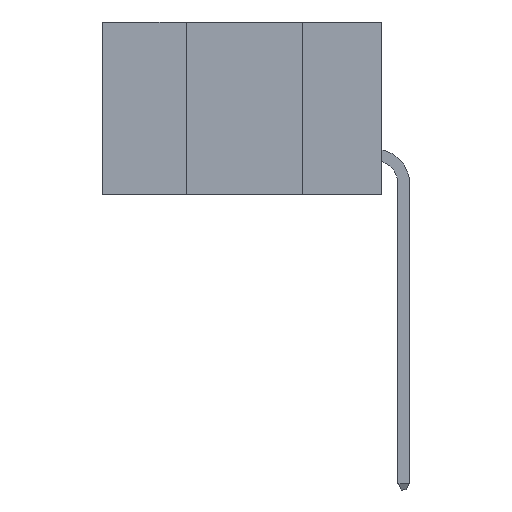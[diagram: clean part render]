
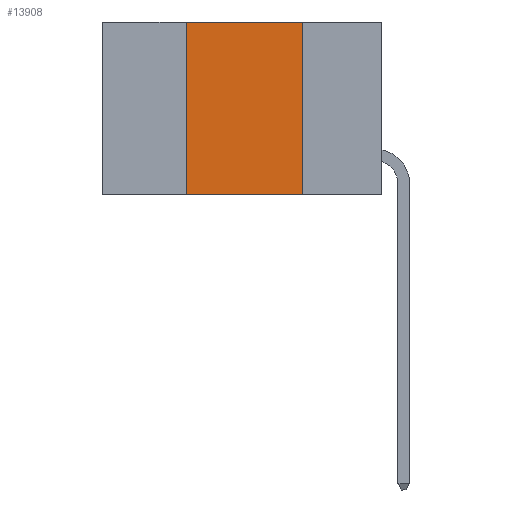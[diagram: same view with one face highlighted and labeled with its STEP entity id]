
A CAD part, left-side view. The second image highlights one B-rep face of the part: STEP entity #13908.
In plain terms, the highlighted planar face has unit normal (-1, 0, 0).
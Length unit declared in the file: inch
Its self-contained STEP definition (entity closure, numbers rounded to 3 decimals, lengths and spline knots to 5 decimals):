
#255 = LINE ( 'NONE', #19461, #16417 ) ;
#271 = EDGE_CURVE ( 'NONE', #3224, #4547, #255, .T. ) ;
#298 = ORIENTED_EDGE ( 'NONE', *, *, #18819, .F. ) ;
#656 = LINE ( 'NONE', #2862, #17238 ) ;
#894 = VERTEX_POINT ( 'NONE', #2922 ) ;
#2625 = AXIS2_PLACEMENT_3D ( 'NONE', #12504, #4800, #15581 ) ;
#2862 = CARTESIAN_POINT ( 'NONE',  ( 0., 0.42, 0. ) ) ;
#2922 = CARTESIAN_POINT ( 'NONE',  ( 0., 0.42, -0.37 ) ) ;
#3003 = DIRECTION ( 'NONE',  ( 0., -1., 0. ) ) ;
#3224 = VERTEX_POINT ( 'NONE', #3853 ) ;
#3259 = CARTESIAN_POINT ( 'NONE',  ( 0., 0.17, -0.37 ) ) ;
#3853 = CARTESIAN_POINT ( 'NONE',  ( 0., 0.42, 0. ) ) ;
#4547 = VERTEX_POINT ( 'NONE', #10092 ) ;
#4800 = DIRECTION ( 'NONE',  ( 1., 0., 0. ) ) ;
#4861 = EDGE_CURVE ( 'NONE', #4547, #14639, #5913, .T. ) ;
#5913 = LINE ( 'NONE', #13743, #10089 ) ;
#7158 = ORIENTED_EDGE ( 'NONE', *, *, #8276, .T. ) ;
#8276 = EDGE_CURVE ( 'NONE', #894, #14639, #17342, .T. ) ;
#9181 = DIRECTION ( 'NONE',  ( 0., 0., -1. ) ) ;
#9233 = ORIENTED_EDGE ( 'NONE', *, *, #4861, .F. ) ;
#9262 = VECTOR ( 'NONE', #3003, 39.37008 ) ;
#9538 = CARTESIAN_POINT ( 'NONE',  ( 0., 0.6, -0.37 ) ) ;
#10089 = VECTOR ( 'NONE', #9181, 39.37008 ) ;
#10092 = CARTESIAN_POINT ( 'NONE',  ( 0., 0.17, 0. ) ) ;
#10672 = ORIENTED_EDGE ( 'NONE', *, *, #271, .F. ) ;
#12504 = CARTESIAN_POINT ( 'NONE',  ( 0., 0.6, 0. ) ) ;
#13743 = CARTESIAN_POINT ( 'NONE',  ( 0., 0.17, 0. ) ) ;
#13744 = DIRECTION ( 'NONE',  ( 0., 0., 1. ) ) ;
#13908 = ADVANCED_FACE ( 'NONE', ( #14584 ), #19980, .F. ) ;
#14584 = FACE_OUTER_BOUND ( 'NONE', #15955, .T. ) ;
#14639 = VERTEX_POINT ( 'NONE', #3259 ) ;
#15581 = DIRECTION ( 'NONE',  ( 0., 0., -1. ) ) ;
#15955 = EDGE_LOOP ( 'NONE', ( #9233, #10672, #298, #7158 ) ) ;
#16417 = VECTOR ( 'NONE', #19844, 39.37008 ) ;
#17238 = VECTOR ( 'NONE', #13744, 39.37008 ) ;
#17342 = LINE ( 'NONE', #9538, #9262 ) ;
#18819 = EDGE_CURVE ( 'NONE', #894, #3224, #656, .T. ) ;
#19461 = CARTESIAN_POINT ( 'NONE',  ( 0., 0.6, 0. ) ) ;
#19844 = DIRECTION ( 'NONE',  ( 0., -1., 0. ) ) ;
#19980 = PLANE ( 'NONE',  #2625 ) ;
